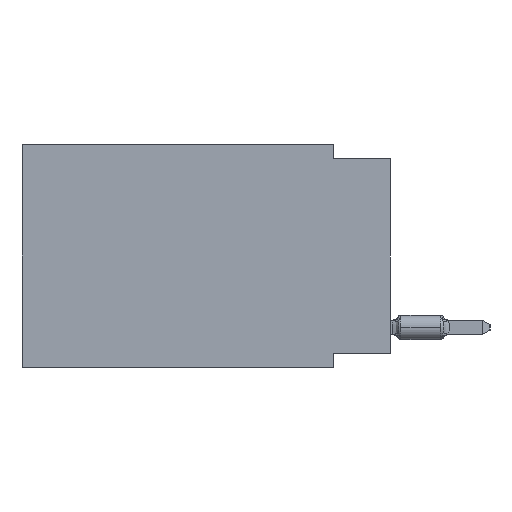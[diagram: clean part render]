
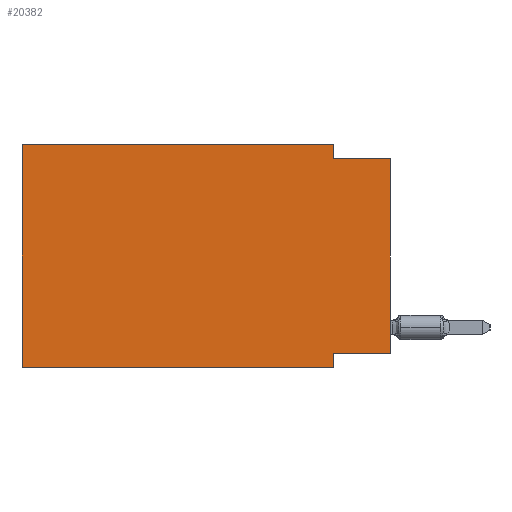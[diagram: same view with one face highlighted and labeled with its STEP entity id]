
A CAD part, left-side view. The second image highlights one B-rep face of the part: STEP entity #20382.
In plain terms, the highlighted planar face has unit normal (-1, 0, 0).
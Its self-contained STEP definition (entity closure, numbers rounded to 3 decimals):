
#693 = CARTESIAN_POINT ( 'NONE',  ( 0., 2.54, -9.271 ) ) ;
#1929 = CARTESIAN_POINT ( 'NONE',  ( 0., 0., -0.635 ) ) ;
#4551 = DIRECTION ( 'NONE',  ( 0., -1., 0. ) ) ;
#5030 = DIRECTION ( 'NONE',  ( 0., 0., -1. ) ) ;
#5150 = LINE ( 'NONE', #18954, #6874 ) ;
#5765 = DIRECTION ( 'NONE',  ( 0., 0., 1. ) ) ;
#5887 = ORIENTED_EDGE ( 'NONE', *, *, #18417, .F. ) ;
#5981 = VERTEX_POINT ( 'NONE', #25273 ) ;
#6806 = EDGE_CURVE ( 'NONE', #27272, #16801, #10830, .T. ) ;
#6874 = VECTOR ( 'NONE', #24490, 1000. ) ;
#7130 = ORIENTED_EDGE ( 'NONE', *, *, #44678, .T. ) ;
#9085 = VERTEX_POINT ( 'NONE', #693 ) ;
#10830 = LINE ( 'NONE', #1929, #24667 ) ;
#13700 = LINE ( 'NONE', #52338, #58886 ) ;
#15912 = ORIENTED_EDGE ( 'NONE', *, *, #57282, .F. ) ;
#16801 = VERTEX_POINT ( 'NONE', #18002 ) ;
#17558 = AXIS2_PLACEMENT_3D ( 'NONE', #26322, #55171, #50567 ) ;
#18002 = CARTESIAN_POINT ( 'NONE',  ( 0., 0., -0.635 ) ) ;
#18417 = EDGE_CURVE ( 'NONE', #35338, #9085, #57095, .T. ) ;
#18689 = ORIENTED_EDGE ( 'NONE', *, *, #39183, .T. ) ;
#18954 = CARTESIAN_POINT ( 'NONE',  ( 0., 16.383, -9.906 ) ) ;
#19039 = LINE ( 'NONE', #37782, #23014 ) ;
#20213 = ORIENTED_EDGE ( 'NONE', *, *, #37513, .F. ) ;
#20382 = ADVANCED_FACE ( 'NONE', ( #21708 ), #54273, .F. ) ;
#20876 = CARTESIAN_POINT ( 'NONE',  ( 0., 16.383, -9.906 ) ) ;
#21576 = EDGE_CURVE ( 'NONE', #59480, #27272, #13700, .T. ) ;
#21685 = VERTEX_POINT ( 'NONE', #29613 ) ;
#21708 = FACE_OUTER_BOUND ( 'NONE', #35554, .T. ) ;
#21887 = DIRECTION ( 'NONE',  ( 0., 0., 1. ) ) ;
#23014 = VECTOR ( 'NONE', #21887, 1000. ) ;
#23129 = LINE ( 'NONE', #47112, #43381 ) ;
#23133 = VECTOR ( 'NONE', #5765, 1000. ) ;
#24362 = ORIENTED_EDGE ( 'NONE', *, *, #31447, .F. ) ;
#24490 = DIRECTION ( 'NONE',  ( 0., -1., 0. ) ) ;
#24667 = VECTOR ( 'NONE', #38486, 1000. ) ;
#25273 = CARTESIAN_POINT ( 'NONE',  ( 0., 2.54, -9.906 ) ) ;
#26271 = VECTOR ( 'NONE', #27613, 1000. ) ;
#26322 = CARTESIAN_POINT ( 'NONE',  ( 0., 16.383, 0. ) ) ;
#27272 = VERTEX_POINT ( 'NONE', #51181 ) ;
#27613 = DIRECTION ( 'NONE',  ( 0., 1., 0. ) ) ;
#29613 = CARTESIAN_POINT ( 'NONE',  ( 0., 16.383, 0. ) ) ;
#30838 = VERTEX_POINT ( 'NONE', #20876 ) ;
#31447 = EDGE_CURVE ( 'NONE', #9085, #5981, #23129, .T. ) ;
#31963 = ORIENTED_EDGE ( 'NONE', *, *, #21576, .F. ) ;
#33715 = LINE ( 'NONE', #47852, #23133 ) ;
#35338 = VERTEX_POINT ( 'NONE', #42496 ) ;
#35554 = EDGE_LOOP ( 'NONE', ( #18689, #41770, #31963, #20213, #15912, #7130, #24362, #5887 ) ) ;
#37513 = EDGE_CURVE ( 'NONE', #21685, #59480, #42328, .T. ) ;
#37782 = CARTESIAN_POINT ( 'NONE',  ( 0., 16.383, 0. ) ) ;
#38486 = DIRECTION ( 'NONE',  ( 0., -1., 0. ) ) ;
#38515 = DIRECTION ( 'NONE',  ( 0., 0., -1. ) ) ;
#39183 = EDGE_CURVE ( 'NONE', #35338, #16801, #33715, .T. ) ;
#41410 = CARTESIAN_POINT ( 'NONE',  ( 0., 16.383, 0. ) ) ;
#41740 = CARTESIAN_POINT ( 'NONE',  ( 0., 0., -9.271 ) ) ;
#41770 = ORIENTED_EDGE ( 'NONE', *, *, #6806, .F. ) ;
#42328 = LINE ( 'NONE', #41410, #50617 ) ;
#42496 = CARTESIAN_POINT ( 'NONE',  ( 0., 0., -9.271 ) ) ;
#43381 = VECTOR ( 'NONE', #5030, 1000. ) ;
#44678 = EDGE_CURVE ( 'NONE', #30838, #5981, #5150, .T. ) ;
#47112 = CARTESIAN_POINT ( 'NONE',  ( 0., 2.54, -9.906 ) ) ;
#47852 = CARTESIAN_POINT ( 'NONE',  ( 0., 0., 0. ) ) ;
#50567 = DIRECTION ( 'NONE',  ( 0., 0., -1. ) ) ;
#50617 = VECTOR ( 'NONE', #4551, 1000. ) ;
#51181 = CARTESIAN_POINT ( 'NONE',  ( 0., 2.54, -0.635 ) ) ;
#52338 = CARTESIAN_POINT ( 'NONE',  ( 0., 2.54, 0. ) ) ;
#54273 = PLANE ( 'NONE',  #17558 ) ;
#55171 = DIRECTION ( 'NONE',  ( 1., 0., 0. ) ) ;
#56797 = CARTESIAN_POINT ( 'NONE',  ( 0., 2.54, 0. ) ) ;
#57095 = LINE ( 'NONE', #41740, #26271 ) ;
#57282 = EDGE_CURVE ( 'NONE', #30838, #21685, #19039, .T. ) ;
#58886 = VECTOR ( 'NONE', #38515, 1000. ) ;
#59480 = VERTEX_POINT ( 'NONE', #56797 ) ;
